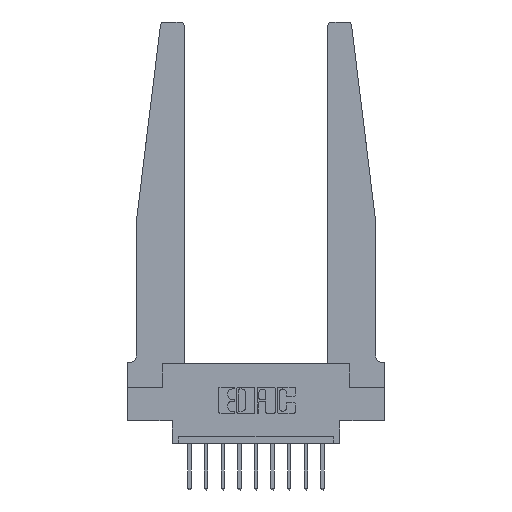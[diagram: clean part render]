
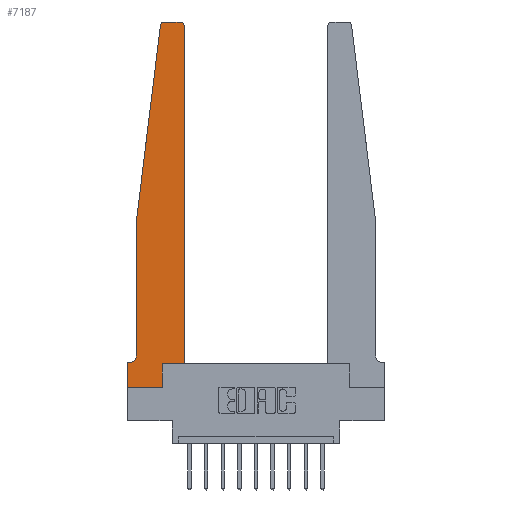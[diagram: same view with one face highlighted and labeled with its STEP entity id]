
A CAD part, top view. The second image highlights one B-rep face of the part: STEP entity #7187.
In plain terms, the highlighted planar face has unit normal (0, 0, 1).
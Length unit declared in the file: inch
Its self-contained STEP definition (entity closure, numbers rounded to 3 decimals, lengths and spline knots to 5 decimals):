
#97 = VERTEX_POINT ( 'NONE', #2744 ) ;
#182 = LINE ( 'NONE', #8407, #12988 ) ;
#558 = CARTESIAN_POINT ( 'NONE',  ( 0.395, 2.75, 0.37 ) ) ;
#776 = CIRCLE ( 'NONE', #9169, 0.03 ) ;
#787 = VERTEX_POINT ( 'NONE', #6341 ) ;
#985 = CIRCLE ( 'NONE', #1986, 0.03 ) ;
#1244 = ORIENTED_EDGE ( 'NONE', *, *, #4130, .T. ) ;
#1367 = AXIS2_PLACEMENT_3D ( 'NONE', #8832, #4202, #11430 ) ;
#1974 = DIRECTION ( 'NONE',  ( 0., 1., 0. ) ) ;
#1986 = AXIS2_PLACEMENT_3D ( 'NONE', #2762, #10969, #7391 ) ;
#2191 = EDGE_CURVE ( 'NONE', #13148, #13645, #985, .T. ) ;
#2383 = VECTOR ( 'NONE', #5754, 39.37008 ) ;
#2490 = VECTOR ( 'NONE', #7091, 39.37008 ) ;
#2744 = CARTESIAN_POINT ( 'NONE',  ( 0., 0.1875, 0.37 ) ) ;
#2762 = CARTESIAN_POINT ( 'NONE',  ( 0.27653, 2.72, 0.37 ) ) ;
#2774 = VECTOR ( 'NONE', #14324, 39.37008 ) ;
#3112 = ORIENTED_EDGE ( 'NONE', *, *, #12812, .T. ) ;
#3160 = ORIENTED_EDGE ( 'NONE', *, *, #6764, .T. ) ;
#3215 = LINE ( 'NONE', #3236, #14778 ) ;
#3236 = CARTESIAN_POINT ( 'NONE',  ( 0.065, 0.1875, 0.37 ) ) ;
#3238 = EDGE_CURVE ( 'NONE', #6774, #6087, #3654, .T. ) ;
#3273 = ORIENTED_EDGE ( 'NONE', *, *, #3238, .T. ) ;
#3302 = CARTESIAN_POINT ( 'NONE',  ( 0.065, 1.25, 0.37 ) ) ;
#3654 = LINE ( 'NONE', #12632, #2383 ) ;
#3825 = CARTESIAN_POINT ( 'NONE',  ( 0.27653, 2.75, 0.37 ) ) ;
#3867 = LINE ( 'NONE', #9772, #2774 ) ;
#3897 = LINE ( 'NONE', #3302, #5524 ) ;
#4011 = VERTEX_POINT ( 'NONE', #558 ) ;
#4041 = EDGE_CURVE ( 'NONE', #14311, #97, #3215, .T. ) ;
#4130 = EDGE_CURVE ( 'NONE', #4011, #13148, #4317, .T. ) ;
#4202 = DIRECTION ( 'NONE',  ( 0., 0., -1. ) ) ;
#4317 = LINE ( 'NONE', #5829, #2490 ) ;
#4511 = CARTESIAN_POINT ( 'NONE',  ( 0.065, 1.25, 0.37 ) ) ;
#4833 = ORIENTED_EDGE ( 'NONE', *, *, #5584, .T. ) ;
#5524 = VECTOR ( 'NONE', #11362, 39.37008 ) ;
#5584 = EDGE_CURVE ( 'NONE', #13645, #12404, #3897, .T. ) ;
#5586 = DIRECTION ( 'NONE',  ( -1., 0., 0. ) ) ;
#5754 = DIRECTION ( 'NONE',  ( 1., 0., 0. ) ) ;
#5829 = CARTESIAN_POINT ( 'NONE',  ( 0.25, 2.75, 0.37 ) ) ;
#6087 = VERTEX_POINT ( 'NONE', #6459 ) ;
#6235 = DIRECTION ( 'NONE',  ( 0., 0., 1. ) ) ;
#6333 = DIRECTION ( 'NONE',  ( 1., 0., 0. ) ) ;
#6341 = CARTESIAN_POINT ( 'NONE',  ( 0., 0., 0.37 ) ) ;
#6459 = CARTESIAN_POINT ( 'NONE',  ( 0.425, 0.18, 0.37 ) ) ;
#6663 = EDGE_CURVE ( 'NONE', #787, #7029, #3867, .T. ) ;
#6701 = CARTESIAN_POINT ( 'NONE',  ( 0.065, 0.2375, 0.37 ) ) ;
#6764 = EDGE_CURVE ( 'NONE', #13807, #14311, #11591, .T. ) ;
#6769 = CARTESIAN_POINT ( 'NONE',  ( 0., 0., 0.37 ) ) ;
#6774 = VERTEX_POINT ( 'NONE', #11088 ) ;
#7029 = VERTEX_POINT ( 'NONE', #12000 ) ;
#7047 = LINE ( 'NONE', #12194, #9543 ) ;
#7091 = DIRECTION ( 'NONE',  ( -1., 0., 0. ) ) ;
#7160 = CARTESIAN_POINT ( 'NONE',  ( 0.24675, 2.72367, 0.37 ) ) ;
#7187 = ADVANCED_FACE ( 'NONE', ( #10860 ), #7543, .T. ) ;
#7302 = LINE ( 'NONE', #8870, #13049 ) ;
#7391 = DIRECTION ( 'NONE',  ( 1., 0., 0. ) ) ;
#7489 = CARTESIAN_POINT ( 'NONE',  ( 0., 0.1875, 0.37 ) ) ;
#7543 = PLANE ( 'NONE',  #14776 ) ;
#7629 = LINE ( 'NONE', #6769, #13549 ) ;
#8407 = CARTESIAN_POINT ( 'NONE',  ( 0.2605, 0.18, 0.37 ) ) ;
#8598 = EDGE_CURVE ( 'NONE', #10220, #4011, #776, .T. ) ;
#8780 = DIRECTION ( 'NONE',  ( 1., 0., 0. ) ) ;
#8782 = EDGE_CURVE ( 'NONE', #97, #787, #7629, .T. ) ;
#8832 = CARTESIAN_POINT ( 'NONE',  ( 0.015, 0.2375, 0.37 ) ) ;
#8870 = CARTESIAN_POINT ( 'NONE',  ( 0.425, 0.18, 0.37 ) ) ;
#9045 = DIRECTION ( 'NONE',  ( 0., -1., 0. ) ) ;
#9169 = AXIS2_PLACEMENT_3D ( 'NONE', #14307, #6235, #6333 ) ;
#9207 = EDGE_LOOP ( 'NONE', ( #1244, #10876, #4833, #14705, #3160, #14382, #13346, #13316, #12466, #3273, #3112, #11144 ) ) ;
#9435 = DIRECTION ( 'NONE',  ( 0., 1., 0. ) ) ;
#9543 = VECTOR ( 'NONE', #9994, 39.37008 ) ;
#9772 = CARTESIAN_POINT ( 'NONE',  ( 0., 0., 0.37 ) ) ;
#9813 = DIRECTION ( 'NONE',  ( 0., 0., 1. ) ) ;
#9994 = DIRECTION ( 'NONE',  ( 0., -1., 0. ) ) ;
#10212 = EDGE_CURVE ( 'NONE', #12404, #13807, #7047, .T. ) ;
#10220 = VERTEX_POINT ( 'NONE', #10974 ) ;
#10654 = CARTESIAN_POINT ( 'NONE',  ( 0.015, 0.1875, 0.37 ) ) ;
#10860 = FACE_OUTER_BOUND ( 'NONE', #9207, .T. ) ;
#10876 = ORIENTED_EDGE ( 'NONE', *, *, #2191, .T. ) ;
#10969 = DIRECTION ( 'NONE',  ( 0., 0., 1. ) ) ;
#10974 = CARTESIAN_POINT ( 'NONE',  ( 0.425, 2.72, 0.37 ) ) ;
#11088 = CARTESIAN_POINT ( 'NONE',  ( 0.2605, 0.18, 0.37 ) ) ;
#11144 = ORIENTED_EDGE ( 'NONE', *, *, #8598, .T. ) ;
#11362 = DIRECTION ( 'NONE',  ( -0.122, -0.992, 0. ) ) ;
#11430 = DIRECTION ( 'NONE',  ( -1., 0., 0. ) ) ;
#11591 = CIRCLE ( 'NONE', #1367, 0.05 ) ;
#12000 = CARTESIAN_POINT ( 'NONE',  ( 0.2605, 0., 0.37 ) ) ;
#12194 = CARTESIAN_POINT ( 'NONE',  ( 0.065, 1.25, 0.37 ) ) ;
#12404 = VERTEX_POINT ( 'NONE', #4511 ) ;
#12466 = ORIENTED_EDGE ( 'NONE', *, *, #14823, .T. ) ;
#12632 = CARTESIAN_POINT ( 'NONE',  ( 0.425, 0.18, 0.37 ) ) ;
#12812 = EDGE_CURVE ( 'NONE', #6087, #10220, #7302, .T. ) ;
#12988 = VECTOR ( 'NONE', #9435, 39.37008 ) ;
#13049 = VECTOR ( 'NONE', #1974, 39.37008 ) ;
#13148 = VERTEX_POINT ( 'NONE', #3825 ) ;
#13316 = ORIENTED_EDGE ( 'NONE', *, *, #6663, .T. ) ;
#13346 = ORIENTED_EDGE ( 'NONE', *, *, #8782, .T. ) ;
#13549 = VECTOR ( 'NONE', #9045, 39.37008 ) ;
#13645 = VERTEX_POINT ( 'NONE', #7160 ) ;
#13807 = VERTEX_POINT ( 'NONE', #6701 ) ;
#14307 = CARTESIAN_POINT ( 'NONE',  ( 0.395, 2.72, 0.37 ) ) ;
#14311 = VERTEX_POINT ( 'NONE', #10654 ) ;
#14324 = DIRECTION ( 'NONE',  ( 1., 0., 0. ) ) ;
#14382 = ORIENTED_EDGE ( 'NONE', *, *, #4041, .T. ) ;
#14705 = ORIENTED_EDGE ( 'NONE', *, *, #10212, .T. ) ;
#14776 = AXIS2_PLACEMENT_3D ( 'NONE', #7489, #9813, #8780 ) ;
#14778 = VECTOR ( 'NONE', #5586, 39.37008 ) ;
#14823 = EDGE_CURVE ( 'NONE', #7029, #6774, #182, .T. ) ;
